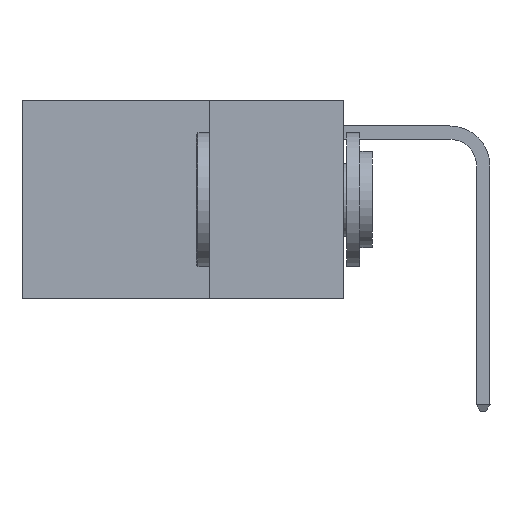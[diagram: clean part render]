
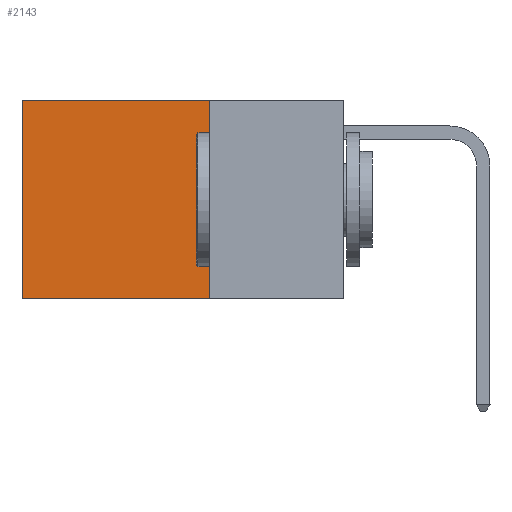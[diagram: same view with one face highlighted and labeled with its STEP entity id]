
A CAD part, left-side view. The second image highlights one B-rep face of the part: STEP entity #2143.
In plain terms, the highlighted planar face has unit normal (-1, 0, 0).
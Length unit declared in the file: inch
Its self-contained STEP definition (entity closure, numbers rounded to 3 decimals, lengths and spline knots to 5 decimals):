
#254 = DIRECTION ( 'NONE',  ( 0., 1., 0. ) ) ;
#667 = LINE ( 'NONE', #6223, #14900 ) ;
#788 = DIRECTION ( 'NONE',  ( 0., 0., -1. ) ) ;
#1309 = CARTESIAN_POINT ( 'NONE',  ( 0.2625, 0.25, -0.37 ) ) ;
#1549 = EDGE_CURVE ( 'NONE', #16288, #11297, #6443, .T. ) ;
#1711 = CARTESIAN_POINT ( 'NONE',  ( 0.2625, 0.25, 0. ) ) ;
#2143 = ADVANCED_FACE ( 'NONE', ( #8317 ), #14614, .F. ) ;
#2849 = CARTESIAN_POINT ( 'NONE',  ( 0.2625, 0.6, 0. ) ) ;
#2994 = DIRECTION ( 'NONE',  ( 0., 0., -1. ) ) ;
#3060 = DIRECTION ( 'NONE',  ( 1., 0., 0. ) ) ;
#4787 = AXIS2_PLACEMENT_3D ( 'NONE', #17058, #3060, #2994 ) ;
#5372 = ORIENTED_EDGE ( 'NONE', *, *, #6878, .T. ) ;
#6040 = EDGE_CURVE ( 'NONE', #11599, #16288, #667, .T. ) ;
#6109 = DIRECTION ( 'NONE',  ( 0., 0., -1. ) ) ;
#6223 = CARTESIAN_POINT ( 'NONE',  ( 0.2625, 0.25, 0. ) ) ;
#6443 = LINE ( 'NONE', #1309, #9603 ) ;
#6878 = EDGE_CURVE ( 'NONE', #11599, #9265, #9761, .T. ) ;
#7375 = EDGE_LOOP ( 'NONE', ( #10662, #10730, #14409, #5372 ) ) ;
#7811 = CARTESIAN_POINT ( 'NONE',  ( 0.2625, 0.25, -0.37 ) ) ;
#8317 = FACE_OUTER_BOUND ( 'NONE', #7375, .T. ) ;
#8656 = DIRECTION ( 'NONE',  ( 0., 1., 0. ) ) ;
#9265 = VERTEX_POINT ( 'NONE', #2849 ) ;
#9603 = VECTOR ( 'NONE', #254, 39.37008 ) ;
#9761 = LINE ( 'NONE', #1711, #12966 ) ;
#10662 = ORIENTED_EDGE ( 'NONE', *, *, #16989, .T. ) ;
#10730 = ORIENTED_EDGE ( 'NONE', *, *, #1549, .F. ) ;
#10935 = CARTESIAN_POINT ( 'NONE',  ( 0.2625, 0.25, 0. ) ) ;
#11297 = VERTEX_POINT ( 'NONE', #17100 ) ;
#11599 = VERTEX_POINT ( 'NONE', #10935 ) ;
#11806 = CARTESIAN_POINT ( 'NONE',  ( 0.2625, 0.6, 0. ) ) ;
#12966 = VECTOR ( 'NONE', #8656, 39.37008 ) ;
#13390 = VECTOR ( 'NONE', #788, 39.37008 ) ;
#14409 = ORIENTED_EDGE ( 'NONE', *, *, #6040, .F. ) ;
#14614 = PLANE ( 'NONE',  #4787 ) ;
#14900 = VECTOR ( 'NONE', #6109, 39.37008 ) ;
#16288 = VERTEX_POINT ( 'NONE', #7811 ) ;
#16989 = EDGE_CURVE ( 'NONE', #9265, #11297, #17372, .T. ) ;
#17058 = CARTESIAN_POINT ( 'NONE',  ( 0.2625, 0.25, 0. ) ) ;
#17100 = CARTESIAN_POINT ( 'NONE',  ( 0.2625, 0.6, -0.37 ) ) ;
#17372 = LINE ( 'NONE', #11806, #13390 ) ;
